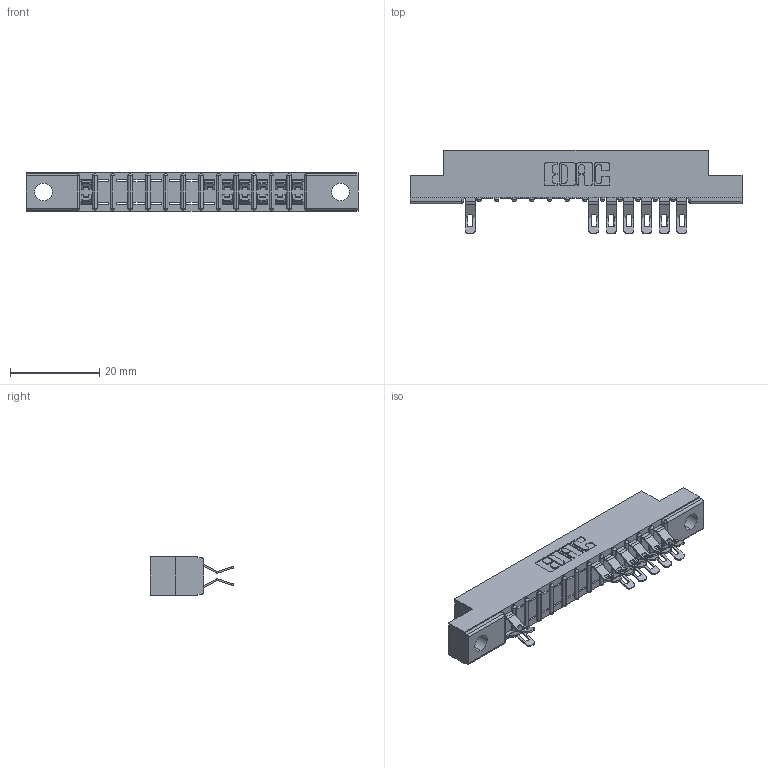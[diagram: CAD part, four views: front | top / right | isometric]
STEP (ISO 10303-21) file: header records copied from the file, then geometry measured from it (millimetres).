
FILE_DESCRIPTION (( 'STEP AP203' ), '1' );
FILE_NAME ('357-026-555-204.STEP', '2018-08-09T03:47:42', ( '' ), ( '' ), 'SwSTEP 2.0', 'SolidWorks 2016', '' );
FILE_SCHEMA (( 'CONFIG_CONTROL_DESIGN' ));
Length unit declared in the file: inch
Products named in the file (3): 307 Part_.156 Dia Mounting Holes; 307-290-001_555; 357-026-555-204
Assembly tree (14 placements, depth 2):
  357-026-555-204
    307 Part_.156 Dia Mounting Holes
    307-290-001_555  x13
Bounding box: 74.52 x 18.75 x 8.71 mm (x, y, z)
Volume: 4640.1 mm3; surface area: 6834.6 mm2
Topology: 14 solids, 14 shells, 1069 faces, 3128 edges, 2028 vertices
Faces by surface type: plane 604, cylinder 437, sphere 28
Entity records: 15675 total; most frequent: CARTESIAN_POINT 2638, ORIENTED_EDGE 2624, DIRECTION 2582, EDGE_CURVE 1312, VECTOR 990, LINE 990, VERTEX_POINT 852, AXIS2_PLACEMENT_3D 796
